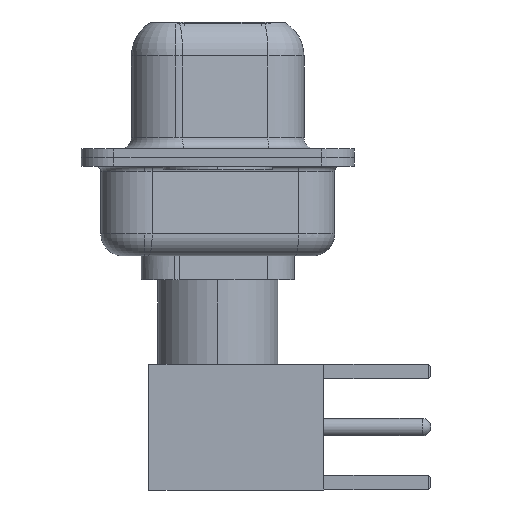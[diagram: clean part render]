
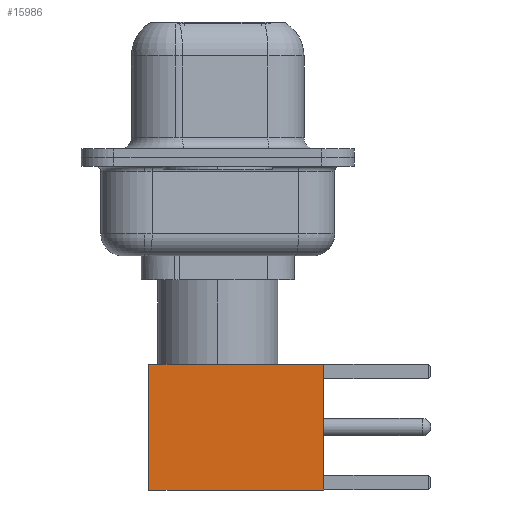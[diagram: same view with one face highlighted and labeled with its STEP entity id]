
A CAD part, left-side view. The second image highlights one B-rep face of the part: STEP entity #15986.
In plain terms, the highlighted face is planar.
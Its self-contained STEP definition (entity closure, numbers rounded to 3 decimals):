
#373 = EDGE_CURVE ( 'NONE', #9562, #12918, #12793, .T. ) ;
#483 = EDGE_LOOP ( 'NONE', ( #11232, #2026, #11832, #10697 ) ) ;
#527 = DIRECTION ( 'NONE',  ( 0., 0., -1. ) ) ;
#612 = VECTOR ( 'NONE', #527, 1000. ) ;
#876 = CARTESIAN_POINT ( 'NONE',  ( 2.875, 2.875, 0. ) ) ;
#884 = VERTEX_POINT ( 'NONE', #12692 ) ;
#992 = VECTOR ( 'NONE', #6333, 1000. ) ;
#2026 = ORIENTED_EDGE ( 'NONE', *, *, #373, .T. ) ;
#2793 = DIRECTION ( 'NONE',  ( 0., 0., 1. ) ) ;
#3068 = EDGE_CURVE ( 'NONE', #6719, #884, #15191, .T. ) ;
#4235 = PLANE ( 'NONE',  #15777 ) ;
#5056 = DIRECTION ( 'NONE',  ( -1., 0., 0. ) ) ;
#5254 = CARTESIAN_POINT ( 'NONE',  ( 2.875, 2.875, 0. ) ) ;
#6177 = CARTESIAN_POINT ( 'NONE',  ( -2.875, 2.875, 0. ) ) ;
#6332 = DIRECTION ( 'NONE',  ( 0., 0., -1. ) ) ;
#6333 = DIRECTION ( 'NONE',  ( -1., 0., 0. ) ) ;
#6719 = VERTEX_POINT ( 'NONE', #13094 ) ;
#7109 = LINE ( 'NONE', #876, #612 ) ;
#7179 = CARTESIAN_POINT ( 'NONE',  ( -2.875, 2.875, 0. ) ) ;
#7504 = CARTESIAN_POINT ( 'NONE',  ( 0., 2.875, 8. ) ) ;
#9562 = VERTEX_POINT ( 'NONE', #10160 ) ;
#9840 = EDGE_CURVE ( 'NONE', #6719, #9562, #7109, .T. ) ;
#10160 = CARTESIAN_POINT ( 'NONE',  ( 2.875, 2.875, 0. ) ) ;
#10255 = CARTESIAN_POINT ( 'NONE',  ( 0., 2.875, 0. ) ) ;
#10385 = FACE_OUTER_BOUND ( 'NONE', #483, .T. ) ;
#10697 = ORIENTED_EDGE ( 'NONE', *, *, #3068, .F. ) ;
#11097 = VECTOR ( 'NONE', #5056, 1000. ) ;
#11232 = ORIENTED_EDGE ( 'NONE', *, *, #9840, .T. ) ;
#11787 = EDGE_CURVE ( 'NONE', #884, #12918, #15266, .T. ) ;
#11832 = ORIENTED_EDGE ( 'NONE', *, *, #11787, .F. ) ;
#12692 = CARTESIAN_POINT ( 'NONE',  ( -2.875, 2.875, 8. ) ) ;
#12793 = LINE ( 'NONE', #10255, #11097 ) ;
#12918 = VERTEX_POINT ( 'NONE', #7179 ) ;
#13094 = CARTESIAN_POINT ( 'NONE',  ( 2.875, 2.875, 8. ) ) ;
#13236 = DIRECTION ( 'NONE',  ( 0., 1., 0. ) ) ;
#15191 = LINE ( 'NONE', #7504, #992 ) ;
#15266 = LINE ( 'NONE', #6177, #15436 ) ;
#15436 = VECTOR ( 'NONE', #6332, 1000. ) ;
#15777 = AXIS2_PLACEMENT_3D ( 'NONE', #5254, #13236, #2793 ) ;
#15986 = ADVANCED_FACE ( 'NONE', ( #10385 ), #4235, .T. ) ;
